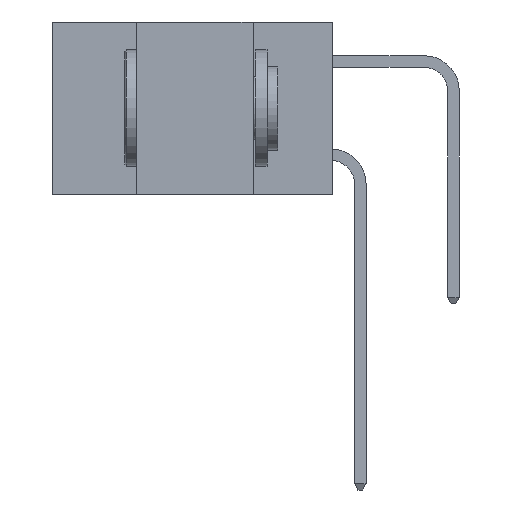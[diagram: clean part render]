
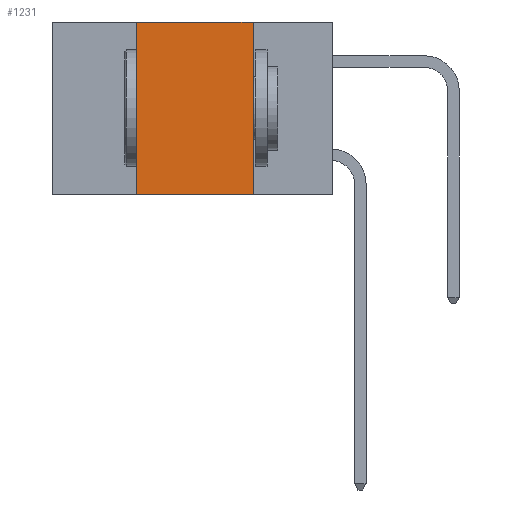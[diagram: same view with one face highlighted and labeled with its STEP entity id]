
A CAD part, left-side view. The second image highlights one B-rep face of the part: STEP entity #1231.
In plain terms, the highlighted planar face has unit normal (-1, 0, 0).
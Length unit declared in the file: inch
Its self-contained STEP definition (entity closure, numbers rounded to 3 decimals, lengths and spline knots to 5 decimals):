
#44 = CARTESIAN_POINT ( 'NONE',  ( 0., 0.6, 0. ) ) ;
#112 = DIRECTION ( 'NONE',  ( 0., -1., 0. ) ) ;
#1073 = VECTOR ( 'NONE', #1079, 39.37008 ) ;
#1079 = DIRECTION ( 'NONE',  ( 0., 0., -1. ) ) ;
#1231 = ADVANCED_FACE ( 'NONE', ( #18208 ), #17128, .F. ) ;
#4126 = VECTOR ( 'NONE', #112, 39.37008 ) ;
#4439 = CARTESIAN_POINT ( 'NONE',  ( 0., 0.17, 0. ) ) ;
#4633 = EDGE_CURVE ( 'NONE', #5320, #18326, #12846, .T. ) ;
#4865 = ORIENTED_EDGE ( 'NONE', *, *, #4633, .F. ) ;
#5320 = VERTEX_POINT ( 'NONE', #4439 ) ;
#5564 = LINE ( 'NONE', #12498, #4126 ) ;
#7725 = EDGE_CURVE ( 'NONE', #14358, #5320, #14412, .T. ) ;
#7957 = VERTEX_POINT ( 'NONE', #10846 ) ;
#8630 = CARTESIAN_POINT ( 'NONE',  ( 0., 0.42, -0.37 ) ) ;
#8737 = EDGE_CURVE ( 'NONE', #7957, #14358, #8925, .T. ) ;
#8925 = LINE ( 'NONE', #8630, #12469 ) ;
#9791 = EDGE_CURVE ( 'NONE', #7957, #18326, #5564, .T. ) ;
#10846 = CARTESIAN_POINT ( 'NONE',  ( 0., 0.42, -0.37 ) ) ;
#10941 = CARTESIAN_POINT ( 'NONE',  ( 0., 0.42, 0. ) ) ;
#11815 = VECTOR ( 'NONE', #13223, 39.37008 ) ;
#12348 = CARTESIAN_POINT ( 'NONE',  ( 0., 0.17, -0.37 ) ) ;
#12469 = VECTOR ( 'NONE', #17684, 39.37008 ) ;
#12477 = ORIENTED_EDGE ( 'NONE', *, *, #7725, .F. ) ;
#12498 = CARTESIAN_POINT ( 'NONE',  ( 0., 0.6, -0.37 ) ) ;
#12600 = ORIENTED_EDGE ( 'NONE', *, *, #8737, .F. ) ;
#12627 = CARTESIAN_POINT ( 'NONE',  ( 0., 0.17, -0.37 ) ) ;
#12846 = LINE ( 'NONE', #12627, #1073 ) ;
#13223 = DIRECTION ( 'NONE',  ( 0., -1., 0. ) ) ;
#13284 = CARTESIAN_POINT ( 'NONE',  ( 0., 0.6, 0. ) ) ;
#14358 = VERTEX_POINT ( 'NONE', #10941 ) ;
#14412 = LINE ( 'NONE', #13284, #11815 ) ;
#14699 = ORIENTED_EDGE ( 'NONE', *, *, #9791, .T. ) ;
#15798 = EDGE_LOOP ( 'NONE', ( #4865, #12477, #12600, #14699 ) ) ;
#17128 = PLANE ( 'NONE',  #17655 ) ;
#17655 = AXIS2_PLACEMENT_3D ( 'NONE', #44, #18265, #18333 ) ;
#17684 = DIRECTION ( 'NONE',  ( 0., 0., 1. ) ) ;
#18208 = FACE_OUTER_BOUND ( 'NONE', #15798, .T. ) ;
#18265 = DIRECTION ( 'NONE',  ( 1., 0., 0. ) ) ;
#18326 = VERTEX_POINT ( 'NONE', #12348 ) ;
#18333 = DIRECTION ( 'NONE',  ( 0., 0., -1. ) ) ;
